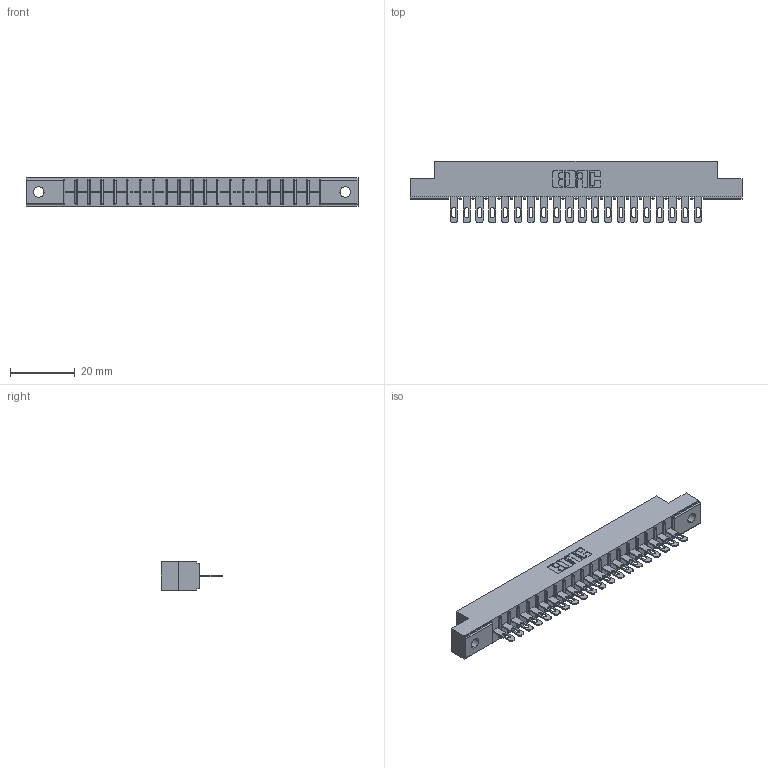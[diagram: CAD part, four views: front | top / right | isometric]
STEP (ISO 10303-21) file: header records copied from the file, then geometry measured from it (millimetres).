
FILE_DESCRIPTION (( 'STEP AP203' ), '1' );
FILE_NAME ('316-020-400-102.STEP', '2020-09-22T19:22:09', ( '' ), ( '' ), 'SwSTEP 2.0', 'SolidWorks 2020', '' );
FILE_SCHEMA (( 'CONFIG_CONTROL_DESIGN' ));
Length unit declared in the file: inch
Products named in the file (3): 306-290-001_100; 316-020-400-102; 306 Part_.128 Dia
Assembly tree (21 placements, depth 2):
  316-020-400-102
    306 Part_.128 Dia
    306-290-001_100  x20
Bounding box: 102.26 x 18.87 x 8.71 mm (x, y, z)
Volume: 7016.6 mm3; surface area: 10358.6 mm2
Topology: 21 solids, 21 shells, 1636 faces, 4616 edges, 2968 vertices
Faces by surface type: plane 1068, cylinder 488, sphere 80
Entity records: 21667 total; most frequent: CARTESIAN_POINT 3635, ORIENTED_EDGE 3600, DIRECTION 3588, EDGE_CURVE 1800, LINE 1394, VECTOR 1394, VERTEX_POINT 1144, AXIS2_PLACEMENT_3D 1097
